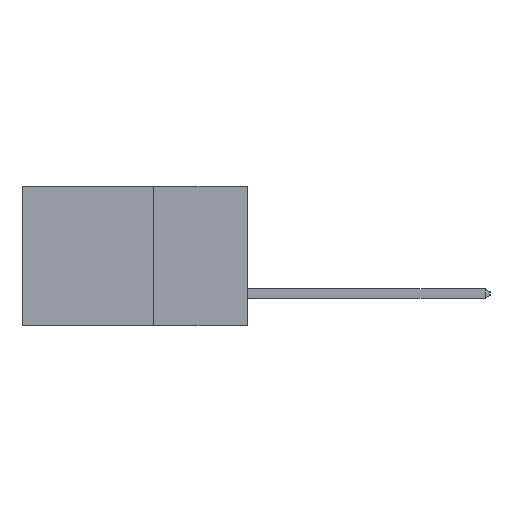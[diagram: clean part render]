
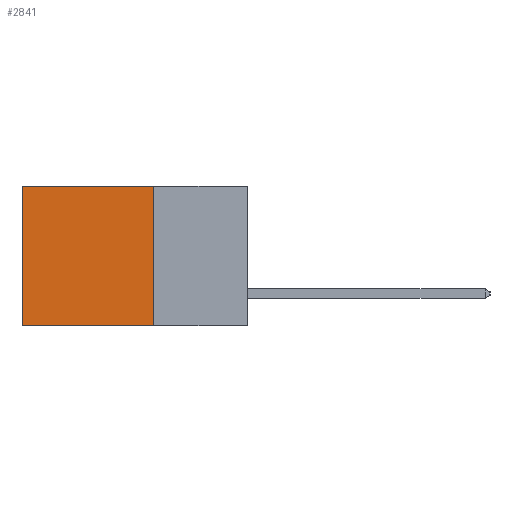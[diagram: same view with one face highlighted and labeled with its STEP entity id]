
A CAD part, left-side view. The second image highlights one B-rep face of the part: STEP entity #2841.
In plain terms, the highlighted planar face has unit normal (-1, 0, 0).
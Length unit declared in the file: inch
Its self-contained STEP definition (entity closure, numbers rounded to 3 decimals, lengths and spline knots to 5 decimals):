
#277 = DIRECTION ( 'NONE',  ( 0., 0., -1. ) ) ;
#544 = CARTESIAN_POINT ( 'NONE',  ( 0.298, 0.6, 0. ) ) ;
#559 = CARTESIAN_POINT ( 'NONE',  ( 0.298, 0.25, 0. ) ) ;
#764 = VERTEX_POINT ( 'NONE', #9149 ) ;
#1296 = VECTOR ( 'NONE', #6654, 39.37008 ) ;
#1369 = CARTESIAN_POINT ( 'NONE',  ( 0.298, 0.6, 0. ) ) ;
#1470 = VERTEX_POINT ( 'NONE', #5231 ) ;
#2206 = EDGE_CURVE ( 'NONE', #1470, #6794, #9183, .T. ) ;
#2518 = AXIS2_PLACEMENT_3D ( 'NONE', #16315, #17665, #9568 ) ;
#2841 = ADVANCED_FACE ( 'NONE', ( #9369 ), #6853, .F. ) ;
#5231 = CARTESIAN_POINT ( 'NONE',  ( 0.298, 0.25, 0. ) ) ;
#5285 = CARTESIAN_POINT ( 'NONE',  ( 0.298, 0.25, -0.37 ) ) ;
#5455 = ORIENTED_EDGE ( 'NONE', *, *, #16199, .T. ) ;
#6427 = LINE ( 'NONE', #1369, #13655 ) ;
#6654 = DIRECTION ( 'NONE',  ( 0., 1., 0. ) ) ;
#6794 = VERTEX_POINT ( 'NONE', #12851 ) ;
#6853 = PLANE ( 'NONE',  #2518 ) ;
#8661 = LINE ( 'NONE', #5285, #1296 ) ;
#9149 = CARTESIAN_POINT ( 'NONE',  ( 0.298, 0.6, -0.37 ) ) ;
#9183 = LINE ( 'NONE', #559, #12375 ) ;
#9369 = FACE_OUTER_BOUND ( 'NONE', #12784, .T. ) ;
#9568 = DIRECTION ( 'NONE',  ( 0., 0., -1. ) ) ;
#10508 = VECTOR ( 'NONE', #12786, 39.37008 ) ;
#10907 = ORIENTED_EDGE ( 'NONE', *, *, #2206, .F. ) ;
#10994 = DIRECTION ( 'NONE',  ( 0., 0., -1. ) ) ;
#11442 = CARTESIAN_POINT ( 'NONE',  ( 0.298, 0.25, 0. ) ) ;
#11801 = EDGE_CURVE ( 'NONE', #12688, #764, #6427, .T. ) ;
#11871 = ORIENTED_EDGE ( 'NONE', *, *, #14221, .F. ) ;
#12375 = VECTOR ( 'NONE', #277, 39.37008 ) ;
#12397 = ORIENTED_EDGE ( 'NONE', *, *, #11801, .T. ) ;
#12688 = VERTEX_POINT ( 'NONE', #544 ) ;
#12784 = EDGE_LOOP ( 'NONE', ( #12397, #11871, #10907, #5455 ) ) ;
#12786 = DIRECTION ( 'NONE',  ( 0., 1., 0. ) ) ;
#12851 = CARTESIAN_POINT ( 'NONE',  ( 0.298, 0.25, -0.37 ) ) ;
#13655 = VECTOR ( 'NONE', #10994, 39.37008 ) ;
#14221 = EDGE_CURVE ( 'NONE', #6794, #764, #8661, .T. ) ;
#14951 = LINE ( 'NONE', #11442, #10508 ) ;
#16199 = EDGE_CURVE ( 'NONE', #1470, #12688, #14951, .T. ) ;
#16315 = CARTESIAN_POINT ( 'NONE',  ( 0.298, 0.25, 0. ) ) ;
#17665 = DIRECTION ( 'NONE',  ( 1., 0., 0. ) ) ;
